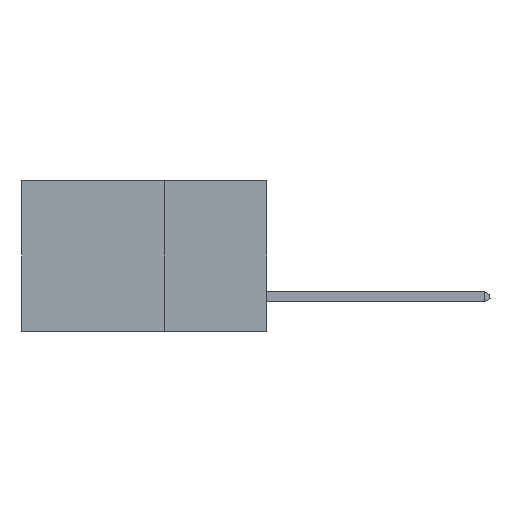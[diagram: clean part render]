
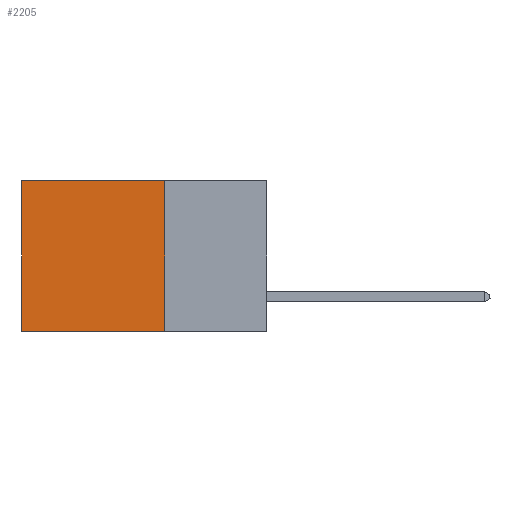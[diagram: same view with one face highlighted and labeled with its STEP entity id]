
A CAD part, left-side view. The second image highlights one B-rep face of the part: STEP entity #2205.
In plain terms, the highlighted planar face has unit normal (-1, 0, 0).
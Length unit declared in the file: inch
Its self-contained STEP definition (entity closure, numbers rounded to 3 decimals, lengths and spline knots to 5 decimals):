
#157 = VERTEX_POINT ( 'NONE', #11134 ) ;
#797 = LINE ( 'NONE', #12775, #11182 ) ;
#1861 = DIRECTION ( 'NONE',  ( 1., 0., 0. ) ) ;
#2205 = ADVANCED_FACE ( 'NONE', ( #2244 ), #4297, .F. ) ;
#2244 = FACE_OUTER_BOUND ( 'NONE', #14981, .T. ) ;
#2709 = DIRECTION ( 'NONE',  ( 0., 1., 0. ) ) ;
#3538 = ORIENTED_EDGE ( 'NONE', *, *, #4864, .T. ) ;
#4297 = PLANE ( 'NONE',  #15504 ) ;
#4864 = EDGE_CURVE ( 'NONE', #10125, #8739, #11358, .T. ) ;
#5394 = EDGE_CURVE ( 'NONE', #157, #9200, #15997, .T. ) ;
#5938 = ORIENTED_EDGE ( 'NONE', *, *, #12341, .F. ) ;
#6893 = DIRECTION ( 'NONE',  ( 0., 0., -1. ) ) ;
#7615 = VECTOR ( 'NONE', #2709, 39.37008 ) ;
#7791 = CARTESIAN_POINT ( 'NONE',  ( 0.2875, 0.25, 0. ) ) ;
#7902 = DIRECTION ( 'NONE',  ( 0., 0., -1. ) ) ;
#8211 = CARTESIAN_POINT ( 'NONE',  ( 0.2875, 0.25, 0. ) ) ;
#8253 = ORIENTED_EDGE ( 'NONE', *, *, #9312, .T. ) ;
#8739 = VERTEX_POINT ( 'NONE', #10593 ) ;
#8966 = VECTOR ( 'NONE', #14034, 39.37008 ) ;
#9200 = VERTEX_POINT ( 'NONE', #14537 ) ;
#9312 = EDGE_CURVE ( 'NONE', #8739, #9200, #14421, .T. ) ;
#9907 = VECTOR ( 'NONE', #15785, 39.37008 ) ;
#10125 = VERTEX_POINT ( 'NONE', #15401 ) ;
#10593 = CARTESIAN_POINT ( 'NONE',  ( 0.2875, 0.6, 0. ) ) ;
#11134 = CARTESIAN_POINT ( 'NONE',  ( 0.2875, 0.25, -0.37 ) ) ;
#11182 = VECTOR ( 'NONE', #7902, 39.37008 ) ;
#11358 = LINE ( 'NONE', #7791, #7615 ) ;
#11895 = ORIENTED_EDGE ( 'NONE', *, *, #5394, .F. ) ;
#12341 = EDGE_CURVE ( 'NONE', #10125, #157, #797, .T. ) ;
#12720 = CARTESIAN_POINT ( 'NONE',  ( 0.2875, 0.25, -0.37 ) ) ;
#12775 = CARTESIAN_POINT ( 'NONE',  ( 0.2875, 0.25, 0. ) ) ;
#12930 = CARTESIAN_POINT ( 'NONE',  ( 0.2875, 0.6, 0. ) ) ;
#14034 = DIRECTION ( 'NONE',  ( 0., 1., 0. ) ) ;
#14421 = LINE ( 'NONE', #12930, #9907 ) ;
#14537 = CARTESIAN_POINT ( 'NONE',  ( 0.2875, 0.6, -0.37 ) ) ;
#14981 = EDGE_LOOP ( 'NONE', ( #8253, #11895, #5938, #3538 ) ) ;
#15401 = CARTESIAN_POINT ( 'NONE',  ( 0.2875, 0.25, 0. ) ) ;
#15504 = AXIS2_PLACEMENT_3D ( 'NONE', #8211, #1861, #6893 ) ;
#15785 = DIRECTION ( 'NONE',  ( 0., 0., -1. ) ) ;
#15997 = LINE ( 'NONE', #12720, #8966 ) ;
